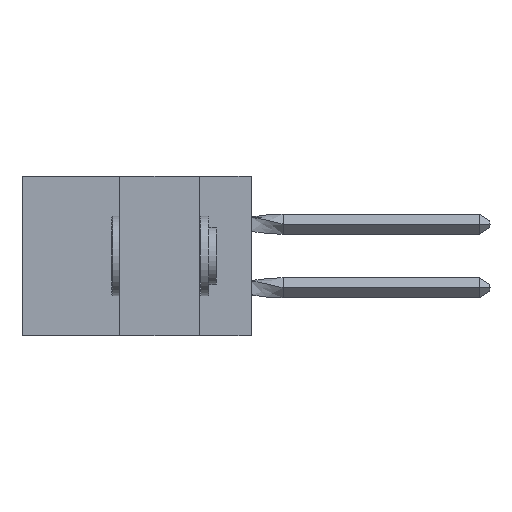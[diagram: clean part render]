
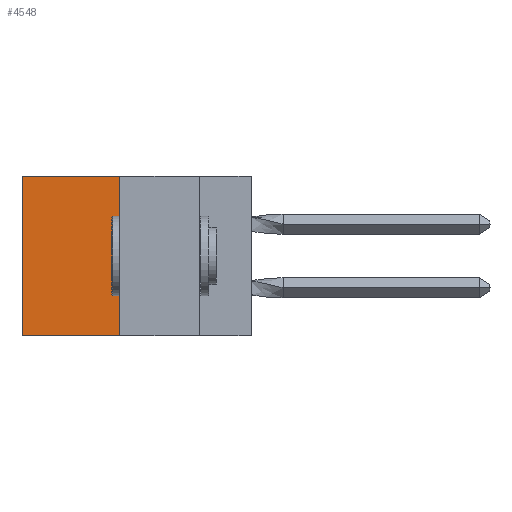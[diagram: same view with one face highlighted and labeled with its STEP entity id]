
A CAD part, left-side view. The second image highlights one B-rep face of the part: STEP entity #4548.
In plain terms, the highlighted planar face has unit normal (-1, 0, 0).
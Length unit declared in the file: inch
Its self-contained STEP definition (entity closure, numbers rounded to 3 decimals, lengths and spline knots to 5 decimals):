
#1065 = DIRECTION ( 'NONE',  ( 0., 1., 0. ) ) ;
#1318 = EDGE_LOOP ( 'NONE', ( #15596, #15096, #15961, #2095 ) ) ;
#1734 = CARTESIAN_POINT ( 'NONE',  ( 0.305, 0.72, -0.5 ) ) ;
#2095 = ORIENTED_EDGE ( 'NONE', *, *, #5939, .T. ) ;
#3418 = DIRECTION ( 'NONE',  ( 0., 0., -1. ) ) ;
#3768 = VERTEX_POINT ( 'NONE', #8698 ) ;
#4548 = ADVANCED_FACE ( 'NONE', ( #6560 ), #14996, .F. ) ;
#4583 = VERTEX_POINT ( 'NONE', #13710 ) ;
#4740 = CARTESIAN_POINT ( 'NONE',  ( 0.305, 0.413, -0.5 ) ) ;
#4914 = CARTESIAN_POINT ( 'NONE',  ( 0.305, 0.413, 0. ) ) ;
#5787 = VECTOR ( 'NONE', #9055, 39.37008 ) ;
#5939 = EDGE_CURVE ( 'NONE', #11007, #4583, #7710, .T. ) ;
#6560 = FACE_OUTER_BOUND ( 'NONE', #1318, .T. ) ;
#6982 = VECTOR ( 'NONE', #9668, 39.37008 ) ;
#7370 = VECTOR ( 'NONE', #3418, 39.37008 ) ;
#7710 = LINE ( 'NONE', #4914, #9220 ) ;
#8619 = CARTESIAN_POINT ( 'NONE',  ( 0.305, 0.413, 0. ) ) ;
#8698 = CARTESIAN_POINT ( 'NONE',  ( 0.305, 0.72, -0.5 ) ) ;
#9055 = DIRECTION ( 'NONE',  ( 0., 0., -1. ) ) ;
#9220 = VECTOR ( 'NONE', #1065, 39.37008 ) ;
#9668 = DIRECTION ( 'NONE',  ( 0., 1., 0. ) ) ;
#9864 = LINE ( 'NONE', #14535, #7370 ) ;
#10268 = DIRECTION ( 'NONE',  ( 1., 0., 0. ) ) ;
#11007 = VERTEX_POINT ( 'NONE', #8619 ) ;
#11370 = CARTESIAN_POINT ( 'NONE',  ( 0.305, 0.413, -0.5 ) ) ;
#11426 = LINE ( 'NONE', #1734, #5787 ) ;
#12544 = DIRECTION ( 'NONE',  ( 0., 0., -1. ) ) ;
#12554 = VERTEX_POINT ( 'NONE', #4740 ) ;
#13505 = EDGE_CURVE ( 'NONE', #11007, #12554, #9864, .T. ) ;
#13710 = CARTESIAN_POINT ( 'NONE',  ( 0.305, 0.72, 0. ) ) ;
#13740 = LINE ( 'NONE', #15763, #6982 ) ;
#14043 = EDGE_CURVE ( 'NONE', #12554, #3768, #13740, .T. ) ;
#14535 = CARTESIAN_POINT ( 'NONE',  ( 0.305, 0.413, -0.5 ) ) ;
#14996 = PLANE ( 'NONE',  #15025 ) ;
#15025 = AXIS2_PLACEMENT_3D ( 'NONE', #11370, #10268, #12544 ) ;
#15093 = EDGE_CURVE ( 'NONE', #4583, #3768, #11426, .T. ) ;
#15096 = ORIENTED_EDGE ( 'NONE', *, *, #14043, .F. ) ;
#15596 = ORIENTED_EDGE ( 'NONE', *, *, #15093, .T. ) ;
#15763 = CARTESIAN_POINT ( 'NONE',  ( 0.305, 0.413, -0.5 ) ) ;
#15961 = ORIENTED_EDGE ( 'NONE', *, *, #13505, .F. ) ;
